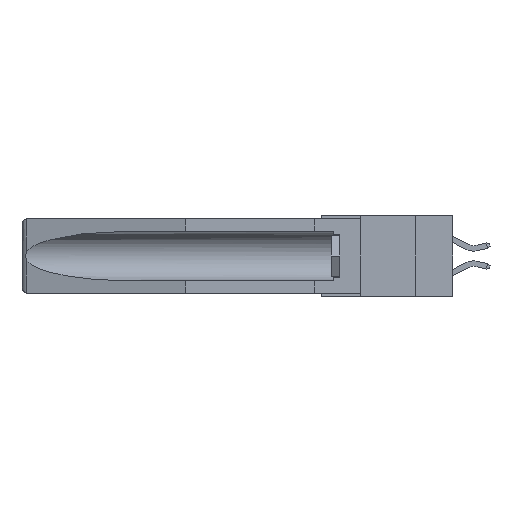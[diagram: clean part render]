
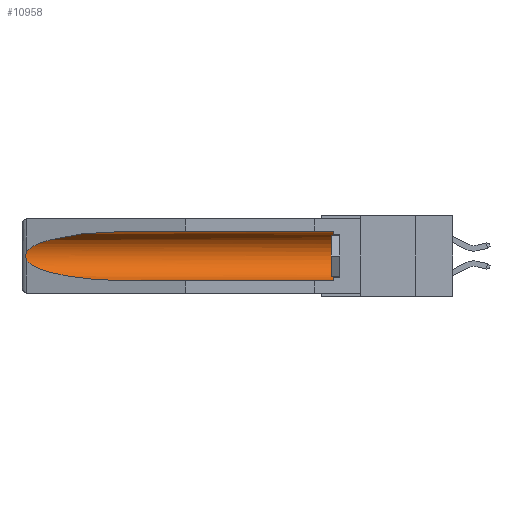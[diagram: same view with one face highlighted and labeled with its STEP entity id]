
A CAD part, left-side view. The second image highlights one B-rep face of the part: STEP entity #10958.
In plain terms, the highlighted cylindrical face has radius 2.857 mm (diameter 5.715 mm), a partial arc.
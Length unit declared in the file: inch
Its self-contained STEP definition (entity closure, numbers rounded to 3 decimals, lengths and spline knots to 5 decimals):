
#355 = CARTESIAN_POINT ( 'NONE',  ( 0.2675, 1.53308, -0.17534 ) ) ;
#446 = ORIENTED_EDGE ( 'NONE', *, *, #16281, .T. ) ;
#659 = CARTESIAN_POINT ( 'NONE',  ( 0.155, -0.30754, -0.059 ) ) ;
#1330 = EDGE_CURVE ( 'NONE', #11136, #4652, #21872, .T. ) ;
#1867 = ORIENTED_EDGE ( 'NONE', *, *, #1330, .T. ) ;
#2656 =( BOUNDED_CURVE ( )  B_SPLINE_CURVE ( 3, ( #4835, #4739, #8778, #25912 ),
 .UNSPECIFIED., .F., .F. ) 
 B_SPLINE_CURVE_WITH_KNOTS ( ( 4, 4 ),
 ( 4.71239, 6.08839 ),
 .UNSPECIFIED. ) 
 CURVE ( )  GEOMETRIC_REPRESENTATION_ITEM ( )  RATIONAL_B_SPLINE_CURVE ( ( 1., 0.848, 0.848, 1. ) ) 
 REPRESENTATION_ITEM ( '' )  );
#3980 = CARTESIAN_POINT ( 'NONE',  ( 0.26537, 1.52718, -0.14972 ) ) ;
#4468 = FACE_OUTER_BOUND ( 'NONE', #19926, .T. ) ;
#4652 = VERTEX_POINT ( 'NONE', #6911 ) ;
#4708 =( BOUNDED_CURVE ( )  B_SPLINE_CURVE ( 3, ( #6133, #12775, #23159, #14819 ),
 .UNSPECIFIED., .F., .F. ) 
 B_SPLINE_CURVE_WITH_KNOTS ( ( 4, 4 ),
 ( 0.1948, 1.5708 ),
 .UNSPECIFIED. ) 
 CURVE ( )  GEOMETRIC_REPRESENTATION_ITEM ( )  RATIONAL_B_SPLINE_CURVE ( ( 1., 0.848, 0.848, 1. ) ) 
 REPRESENTATION_ITEM ( '' )  );
#4739 = CARTESIAN_POINT ( 'NONE',  ( 0.21114, 1.30732, -0.059 ) ) ;
#4744 = CARTESIAN_POINT ( 'NONE',  ( 0.155, -0.30754, -0.1715 ) ) ;
#4759 = CARTESIAN_POINT ( 'NONE',  ( 0.2675, 1.53308, -0.16763 ) ) ;
#4835 = CARTESIAN_POINT ( 'NONE',  ( 0.155, 1.07973, -0.059 ) ) ;
#4857 = CARTESIAN_POINT ( 'NONE',  ( 0.26654, 1.53092, -0.15636 ) ) ;
#5125 = DIRECTION ( 'NONE',  ( 0., 1., 0. ) ) ;
#5178 = ORIENTED_EDGE ( 'NONE', *, *, #8143, .T. ) ;
#5271 = CARTESIAN_POINT ( 'NONE',  ( 0.155, 0.126, -0.1715 ) ) ;
#6133 = CARTESIAN_POINT ( 'NONE',  ( 0.26537, 1.52718, -0.19328 ) ) ;
#6225 = VERTEX_POINT ( 'NONE', #3980 ) ;
#6902 = CARTESIAN_POINT ( 'NONE',  ( 0.26655, 1.53094, -0.18657 ) ) ;
#6911 = CARTESIAN_POINT ( 'NONE',  ( 0.155, 1.07973, -0.059 ) ) ;
#8077 = VERTEX_POINT ( 'NONE', #8737 ) ;
#8143 = EDGE_CURVE ( 'NONE', #8077, #11136, #18659, .T. ) ;
#8616 = EDGE_CURVE ( 'NONE', #6225, #13979, #25401, .T. ) ;
#8737 = CARTESIAN_POINT ( 'NONE',  ( 0.155, 0.126, -0.284 ) ) ;
#8778 = CARTESIAN_POINT ( 'NONE',  ( 0.25451, 1.48313, -0.09465 ) ) ;
#8874 = DIRECTION ( 'NONE',  ( 0., 0., 1. ) ) ;
#8984 = CARTESIAN_POINT ( 'NONE',  ( 0.26537, 1.52718, -0.14972 ) ) ;
#9068 = CARTESIAN_POINT ( 'NONE',  ( 0.26597, 1.5296, -0.19026 ) ) ;
#9128 = LINE ( 'NONE', #26393, #23172 ) ;
#9853 = CYLINDRICAL_SURFACE ( 'NONE', #23739, 0.1125 ) ;
#10137 = ORIENTED_EDGE ( 'NONE', *, *, #11885, .T. ) ;
#10310 = CARTESIAN_POINT ( 'NONE',  ( 0.155, 1.07973, -0.284 ) ) ;
#10958 = ADVANCED_FACE ( 'NONE', ( #4468 ), #9853, .F. ) ;
#11136 = VERTEX_POINT ( 'NONE', #16302 ) ;
#11885 = EDGE_CURVE ( 'NONE', #13979, #25672, #4708, .T. ) ;
#12775 = CARTESIAN_POINT ( 'NONE',  ( 0.25451, 1.48313, -0.24835 ) ) ;
#13354 = CARTESIAN_POINT ( 'NONE',  ( 0.26537, 1.52718, -0.19328 ) ) ;
#13763 = DIRECTION ( 'NONE',  ( 0., 0., 1. ) ) ;
#13979 = VERTEX_POINT ( 'NONE', #19031 ) ;
#14819 = CARTESIAN_POINT ( 'NONE',  ( 0.155, 1.07973, -0.284 ) ) ;
#15059 = ORIENTED_EDGE ( 'NONE', *, *, #8616, .T. ) ;
#16281 = EDGE_CURVE ( 'NONE', #4652, #6225, #2656, .T. ) ;
#16302 = CARTESIAN_POINT ( 'NONE',  ( 0.155, 0.126, -0.059 ) ) ;
#16447 = EDGE_CURVE ( 'NONE', #8077, #25672, #9128, .T. ) ;
#18659 = CIRCLE ( 'NONE', #27577, 0.1125 ) ;
#19031 = CARTESIAN_POINT ( 'NONE',  ( 0.26537, 1.52718, -0.19328 ) ) ;
#19541 = VECTOR ( 'NONE', #24219, 39.37008 ) ;
#19721 = CARTESIAN_POINT ( 'NONE',  ( 0.2673, 1.53269, -0.17917 ) ) ;
#19813 = CARTESIAN_POINT ( 'NONE',  ( 0.2673, 1.5327, -0.16383 ) ) ;
#19926 = EDGE_LOOP ( 'NONE', ( #446, #15059, #10137, #24063, #5178, #1867 ) ) ;
#21841 = DIRECTION ( 'NONE',  ( 0., 1., 0. ) ) ;
#21872 = LINE ( 'NONE', #659, #19541 ) ;
#23159 = CARTESIAN_POINT ( 'NONE',  ( 0.21114, 1.30732, -0.284 ) ) ;
#23172 = VECTOR ( 'NONE', #5125, 39.37008 ) ;
#23739 = AXIS2_PLACEMENT_3D ( 'NONE', #4744, #21841, #8874 ) ;
#24063 = ORIENTED_EDGE ( 'NONE', *, *, #16447, .F. ) ;
#24219 = DIRECTION ( 'NONE',  ( 0., 1., 0. ) ) ;
#25401 = B_SPLINE_CURVE_WITH_KNOTS ( 'NONE', 3,
 ( #8984, #26317, #4857, #19813, #4759, #355, #19721, #6902, #9068, #13354 ),
 .UNSPECIFIED., .F., .F.,
 ( 4, 2, 2, 2, 4 ),
 ( 0., 0.00029, 0.00058, 0.00087, 0.00117 ),
 .UNSPECIFIED. ) ;
#25672 = VERTEX_POINT ( 'NONE', #10310 ) ;
#25912 = CARTESIAN_POINT ( 'NONE',  ( 0.26537, 1.52718, -0.14972 ) ) ;
#26317 = CARTESIAN_POINT ( 'NONE',  ( 0.26597, 1.52961, -0.15275 ) ) ;
#26393 = CARTESIAN_POINT ( 'NONE',  ( 0.155, -0.30754, -0.284 ) ) ;
#26616 = DIRECTION ( 'NONE',  ( 0., -1., 0. ) ) ;
#27577 = AXIS2_PLACEMENT_3D ( 'NONE', #5271, #26616, #13763 ) ;
